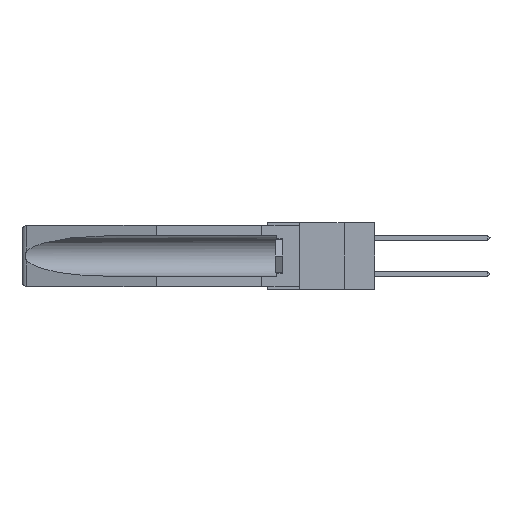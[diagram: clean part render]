
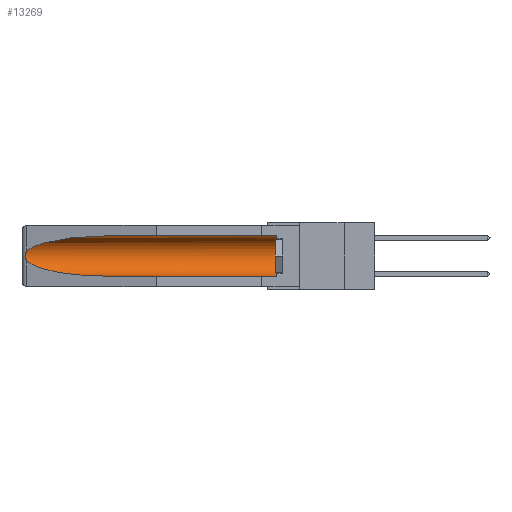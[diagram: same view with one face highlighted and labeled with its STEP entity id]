
A CAD part, left-side view. The second image highlights one B-rep face of the part: STEP entity #13269.
In plain terms, the highlighted cylindrical face has radius 2.857 mm (diameter 5.715 mm), a partial arc.
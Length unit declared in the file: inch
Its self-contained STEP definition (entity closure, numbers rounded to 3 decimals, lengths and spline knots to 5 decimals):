
#206 = EDGE_LOOP ( 'NONE', ( #19928, #12773, #23250, #19409, #16672, #3947 ) ) ;
#373 = CARTESIAN_POINT ( 'NONE',  ( 0.155, 0.126, -0.1715 ) ) ;
#392 = CARTESIAN_POINT ( 'NONE',  ( 0.26537, 1.52718, -0.19328 ) ) ;
#1119 = CARTESIAN_POINT ( 'NONE',  ( 0.155, 1.07973, -0.059 ) ) ;
#1509 = LINE ( 'NONE', #22981, #17296 ) ;
#1773 = CARTESIAN_POINT ( 'NONE',  ( 0.26655, 1.53094, -0.18657 ) ) ;
#2037 = CARTESIAN_POINT ( 'NONE',  ( 0.2675, 1.53308, -0.17534 ) ) ;
#2057 = EDGE_CURVE ( 'NONE', #20991, #5543, #8686, .T. ) ;
#2180 = CARTESIAN_POINT ( 'NONE',  ( 0.155, 0.126, -0.059 ) ) ;
#2381 = DIRECTION ( 'NONE',  ( 0., 0., 1. ) ) ;
#2855 = DIRECTION ( 'NONE',  ( 0., 1., 0. ) ) ;
#3947 = ORIENTED_EDGE ( 'NONE', *, *, #14252, .T. ) ;
#3972 = B_SPLINE_CURVE_WITH_KNOTS ( 'NONE', 3,
 ( #14266, #14181, #6057, #6151, #23977, #2037, #4130, #1773, #20274, #5982 ),
 .UNSPECIFIED., .F., .F.,
 ( 4, 2, 2, 2, 4 ),
 ( 0., 0.00029, 0.00058, 0.00087, 0.00117 ),
 .UNSPECIFIED. ) ;
#4130 = CARTESIAN_POINT ( 'NONE',  ( 0.2673, 1.53269, -0.17917 ) ) ;
#4440 =( BOUNDED_CURVE ( )  B_SPLINE_CURVE ( 3, ( #392, #14614, #22843, #16864 ),
 .UNSPECIFIED., .F., .T. ) 
 B_SPLINE_CURVE_WITH_KNOTS ( ( 4, 4 ),
 ( 0.1948, 1.5708 ),
 .UNSPECIFIED. ) 
 CURVE ( )  GEOMETRIC_REPRESENTATION_ITEM ( )  RATIONAL_B_SPLINE_CURVE ( ( 1., 0.848, 0.848, 1. ) ) 
 REPRESENTATION_ITEM ( '' )  );
#4794 = DIRECTION ( 'NONE',  ( 0., 1., 0. ) ) ;
#5082 = AXIS2_PLACEMENT_3D ( 'NONE', #12761, #4794, #18845 ) ;
#5543 = VERTEX_POINT ( 'NONE', #14189 ) ;
#5982 = CARTESIAN_POINT ( 'NONE',  ( 0.26537, 1.52718, -0.19328 ) ) ;
#6057 = CARTESIAN_POINT ( 'NONE',  ( 0.26654, 1.53092, -0.15636 ) ) ;
#6151 = CARTESIAN_POINT ( 'NONE',  ( 0.2673, 1.5327, -0.16383 ) ) ;
#8686 =( BOUNDED_CURVE ( )  B_SPLINE_CURVE ( 3, ( #1119, #11313, #17181, #23234 ),
 .UNSPECIFIED., .F., .F. ) 
 B_SPLINE_CURVE_WITH_KNOTS ( ( 4, 4 ),
 ( 4.71239, 6.08839 ),
 .UNSPECIFIED. ) 
 CURVE ( )  GEOMETRIC_REPRESENTATION_ITEM ( )  RATIONAL_B_SPLINE_CURVE ( ( 1., 0.848, 0.848, 1. ) ) 
 REPRESENTATION_ITEM ( '' )  );
#10328 = EDGE_CURVE ( 'NONE', #12870, #16280, #15646, .T. ) ;
#10824 = CARTESIAN_POINT ( 'NONE',  ( 0.155, -0.30754, -0.284 ) ) ;
#11229 = CARTESIAN_POINT ( 'NONE',  ( 0.155, 1.07973, -0.059 ) ) ;
#11313 = CARTESIAN_POINT ( 'NONE',  ( 0.21114, 1.30732, -0.059 ) ) ;
#12119 = EDGE_CURVE ( 'NONE', #5543, #15752, #3972, .T. ) ;
#12761 = CARTESIAN_POINT ( 'NONE',  ( 0.155, -0.30754, -0.1715 ) ) ;
#12773 = ORIENTED_EDGE ( 'NONE', *, *, #12119, .T. ) ;
#12870 = VERTEX_POINT ( 'NONE', #19235 ) ;
#13269 = ADVANCED_FACE ( 'NONE', ( #16431 ), #17680, .F. ) ;
#14181 = CARTESIAN_POINT ( 'NONE',  ( 0.26597, 1.52961, -0.15275 ) ) ;
#14189 = CARTESIAN_POINT ( 'NONE',  ( 0.26537, 1.52718, -0.14972 ) ) ;
#14252 = EDGE_CURVE ( 'NONE', #16280, #20991, #1509, .T. ) ;
#14266 = CARTESIAN_POINT ( 'NONE',  ( 0.26537, 1.52718, -0.14972 ) ) ;
#14520 = DIRECTION ( 'NONE',  ( 0., -1., 0. ) ) ;
#14614 = CARTESIAN_POINT ( 'NONE',  ( 0.25451, 1.48313, -0.24835 ) ) ;
#14662 = EDGE_CURVE ( 'NONE', #15752, #24245, #4440, .T. ) ;
#15646 = CIRCLE ( 'NONE', #19677, 0.1125 ) ;
#15752 = VERTEX_POINT ( 'NONE', #24925 ) ;
#16280 = VERTEX_POINT ( 'NONE', #2180 ) ;
#16431 = FACE_OUTER_BOUND ( 'NONE', #206, .T. ) ;
#16672 = ORIENTED_EDGE ( 'NONE', *, *, #10328, .T. ) ;
#16864 = CARTESIAN_POINT ( 'NONE',  ( 0.155, 1.07973, -0.284 ) ) ;
#17181 = CARTESIAN_POINT ( 'NONE',  ( 0.25451, 1.48313, -0.09465 ) ) ;
#17296 = VECTOR ( 'NONE', #2855, 39.37008 ) ;
#17680 = CYLINDRICAL_SURFACE ( 'NONE', #5082, 0.1125 ) ;
#18845 = DIRECTION ( 'NONE',  ( 0., 0., 1. ) ) ;
#19235 = CARTESIAN_POINT ( 'NONE',  ( 0.155, 0.126, -0.284 ) ) ;
#19409 = ORIENTED_EDGE ( 'NONE', *, *, #20203, .F. ) ;
#19677 = AXIS2_PLACEMENT_3D ( 'NONE', #373, #14520, #2381 ) ;
#19928 = ORIENTED_EDGE ( 'NONE', *, *, #2057, .T. ) ;
#19935 = CARTESIAN_POINT ( 'NONE',  ( 0.155, 1.07973, -0.284 ) ) ;
#20198 = VECTOR ( 'NONE', #21059, 39.37008 ) ;
#20203 = EDGE_CURVE ( 'NONE', #12870, #24245, #20829, .T. ) ;
#20274 = CARTESIAN_POINT ( 'NONE',  ( 0.26597, 1.5296, -0.19026 ) ) ;
#20829 = LINE ( 'NONE', #10824, #20198 ) ;
#20991 = VERTEX_POINT ( 'NONE', #11229 ) ;
#21059 = DIRECTION ( 'NONE',  ( 0., 1., 0. ) ) ;
#22843 = CARTESIAN_POINT ( 'NONE',  ( 0.21114, 1.30732, -0.284 ) ) ;
#22981 = CARTESIAN_POINT ( 'NONE',  ( 0.155, -0.30754, -0.059 ) ) ;
#23234 = CARTESIAN_POINT ( 'NONE',  ( 0.26537, 1.52718, -0.14972 ) ) ;
#23250 = ORIENTED_EDGE ( 'NONE', *, *, #14662, .T. ) ;
#23977 = CARTESIAN_POINT ( 'NONE',  ( 0.2675, 1.53308, -0.16763 ) ) ;
#24245 = VERTEX_POINT ( 'NONE', #19935 ) ;
#24925 = CARTESIAN_POINT ( 'NONE',  ( 0.26537, 1.52718, -0.19328 ) ) ;
